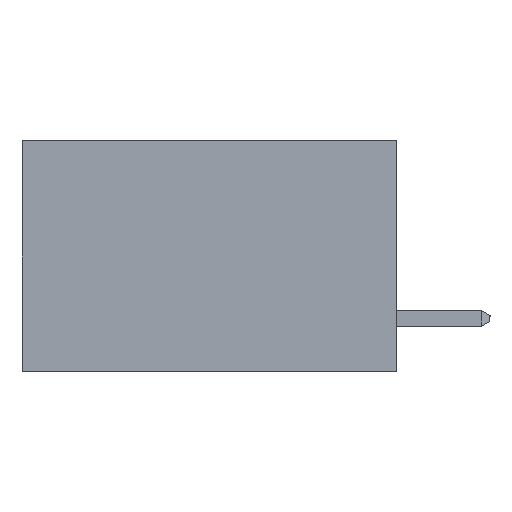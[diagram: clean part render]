
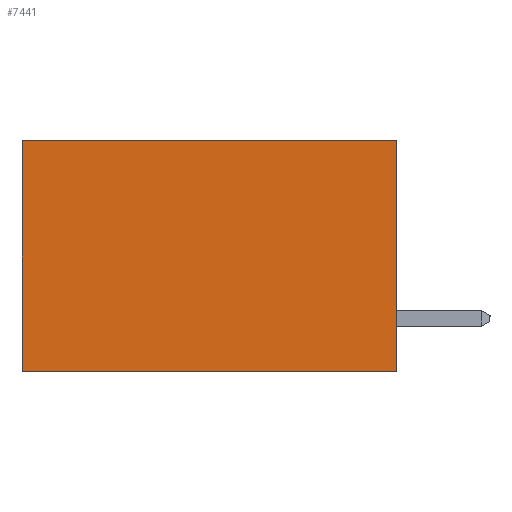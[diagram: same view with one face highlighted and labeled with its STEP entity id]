
A CAD part, left-side view. The second image highlights one B-rep face of the part: STEP entity #7441.
In plain terms, the highlighted planar face has unit normal (-1, 0, 0).
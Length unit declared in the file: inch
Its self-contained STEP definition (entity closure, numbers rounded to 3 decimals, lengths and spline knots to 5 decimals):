
#272 = LINE ( 'NONE', #9189, #16410 ) ;
#1695 = EDGE_LOOP ( 'NONE', ( #19229, #19369, #11965, #18320 ) ) ;
#1780 = VERTEX_POINT ( 'NONE', #4191 ) ;
#1908 = LINE ( 'NONE', #16570, #9747 ) ;
#2215 = EDGE_CURVE ( 'NONE', #1780, #7244, #2771, .T. ) ;
#2277 = VECTOR ( 'NONE', #3195, 39.37008 ) ;
#2604 = CARTESIAN_POINT ( 'NONE',  ( 0.2615, 0., -0.37 ) ) ;
#2771 = LINE ( 'NONE', #4617, #2277 ) ;
#3195 = DIRECTION ( 'NONE',  ( 0., 1., 0. ) ) ;
#3299 = DIRECTION ( 'NONE',  ( 0., 0., -1. ) ) ;
#3622 = CARTESIAN_POINT ( 'NONE',  ( 0.2615, 0.6, 0. ) ) ;
#3977 = EDGE_CURVE ( 'NONE', #7244, #14812, #272, .T. ) ;
#4162 = DIRECTION ( 'NONE',  ( 0., 0., -1. ) ) ;
#4191 = CARTESIAN_POINT ( 'NONE',  ( 0.2615, 0., 0. ) ) ;
#4496 = CARTESIAN_POINT ( 'NONE',  ( 0.2615, 0., -0.37 ) ) ;
#4617 = CARTESIAN_POINT ( 'NONE',  ( 0.2615, 0., 0. ) ) ;
#6247 = VERTEX_POINT ( 'NONE', #12159 ) ;
#7244 = VERTEX_POINT ( 'NONE', #3622 ) ;
#7441 = ADVANCED_FACE ( 'NONE', ( #13270 ), #19685, .F. ) ;
#9189 = CARTESIAN_POINT ( 'NONE',  ( 0.2615, 0.6, -0.37 ) ) ;
#9747 = VECTOR ( 'NONE', #18088, 39.37008 ) ;
#11845 = VECTOR ( 'NONE', #13945, 39.37008 ) ;
#11965 = ORIENTED_EDGE ( 'NONE', *, *, #13741, .F. ) ;
#12159 = CARTESIAN_POINT ( 'NONE',  ( 0.2615, 0., -0.37 ) ) ;
#12966 = AXIS2_PLACEMENT_3D ( 'NONE', #2604, #13611, #4162 ) ;
#13270 = FACE_OUTER_BOUND ( 'NONE', #1695, .T. ) ;
#13611 = DIRECTION ( 'NONE',  ( 1., 0., 0. ) ) ;
#13741 = EDGE_CURVE ( 'NONE', #1780, #6247, #1908, .T. ) ;
#13945 = DIRECTION ( 'NONE',  ( 0., 1., 0. ) ) ;
#14436 = CARTESIAN_POINT ( 'NONE',  ( 0.2615, 0.6, -0.37 ) ) ;
#14812 = VERTEX_POINT ( 'NONE', #14436 ) ;
#16410 = VECTOR ( 'NONE', #3299, 39.37008 ) ;
#16570 = CARTESIAN_POINT ( 'NONE',  ( 0.2615, 0., -0.37 ) ) ;
#16958 = EDGE_CURVE ( 'NONE', #6247, #14812, #20042, .T. ) ;
#18088 = DIRECTION ( 'NONE',  ( 0., 0., -1. ) ) ;
#18320 = ORIENTED_EDGE ( 'NONE', *, *, #2215, .T. ) ;
#19229 = ORIENTED_EDGE ( 'NONE', *, *, #3977, .T. ) ;
#19369 = ORIENTED_EDGE ( 'NONE', *, *, #16958, .F. ) ;
#19685 = PLANE ( 'NONE',  #12966 ) ;
#20042 = LINE ( 'NONE', #4496, #11845 ) ;
